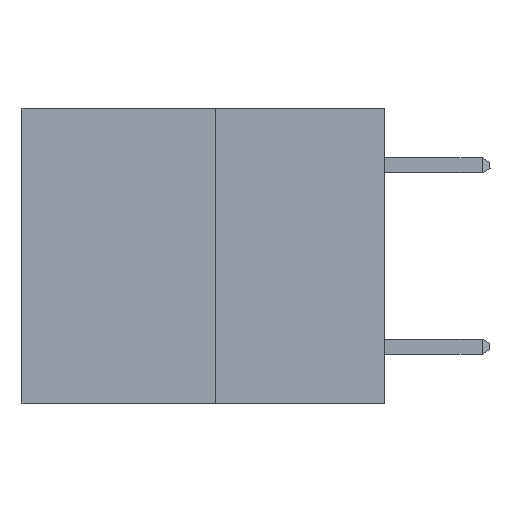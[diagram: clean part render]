
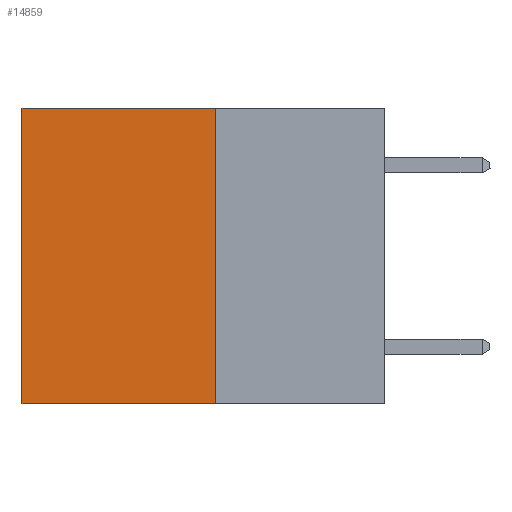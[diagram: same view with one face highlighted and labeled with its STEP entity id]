
A CAD part, left-side view. The second image highlights one B-rep face of the part: STEP entity #14859.
In plain terms, the highlighted planar face has unit normal (-1, 0, 0).
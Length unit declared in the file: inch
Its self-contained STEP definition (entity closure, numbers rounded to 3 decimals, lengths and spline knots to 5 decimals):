
#850 = DIRECTION ( 'NONE',  ( 0., 1., 0. ) ) ;
#1541 = LINE ( 'NONE', #23068, #5749 ) ;
#2603 = VECTOR ( 'NONE', #850, 39.37008 ) ;
#3437 = ORIENTED_EDGE ( 'NONE', *, *, #22030, .F. ) ;
#4077 = VECTOR ( 'NONE', #6799, 39.37008 ) ;
#4344 = VERTEX_POINT ( 'NONE', #21562 ) ;
#5150 = DIRECTION ( 'NONE',  ( 0., 0., -1. ) ) ;
#5749 = VECTOR ( 'NONE', #22993, 39.37008 ) ;
#6559 = CARTESIAN_POINT ( 'NONE',  ( 0.3165, 0.28, -0.49 ) ) ;
#6799 = DIRECTION ( 'NONE',  ( 0., 0., -1. ) ) ;
#6869 = FACE_OUTER_BOUND ( 'NONE', #19463, .T. ) ;
#7424 = AXIS2_PLACEMENT_3D ( 'NONE', #11997, #17284, #8330 ) ;
#7806 = VERTEX_POINT ( 'NONE', #21956 ) ;
#8330 = DIRECTION ( 'NONE',  ( 0., 0., -1. ) ) ;
#9907 = CARTESIAN_POINT ( 'NONE',  ( 0.3165, 0.6, -0.49 ) ) ;
#9951 = CARTESIAN_POINT ( 'NONE',  ( 0.3165, 0.6, 0. ) ) ;
#11497 = ORIENTED_EDGE ( 'NONE', *, *, #23330, .T. ) ;
#11788 = CARTESIAN_POINT ( 'NONE',  ( 0.3165, 0.28, -0.49 ) ) ;
#11997 = CARTESIAN_POINT ( 'NONE',  ( 0.3165, 0.28, -0.49 ) ) ;
#12195 = VERTEX_POINT ( 'NONE', #9951 ) ;
#12537 = ORIENTED_EDGE ( 'NONE', *, *, #13540, .T. ) ;
#13540 = EDGE_CURVE ( 'NONE', #4344, #12195, #1541, .T. ) ;
#14174 = LINE ( 'NONE', #11788, #2603 ) ;
#14859 = ADVANCED_FACE ( 'NONE', ( #6869 ), #17208, .F. ) ;
#16576 = CARTESIAN_POINT ( 'NONE',  ( 0.3165, 0.6, -0.49 ) ) ;
#17044 = ORIENTED_EDGE ( 'NONE', *, *, #20239, .F. ) ;
#17208 = PLANE ( 'NONE',  #7424 ) ;
#17284 = DIRECTION ( 'NONE',  ( 1., 0., 0. ) ) ;
#19463 = EDGE_LOOP ( 'NONE', ( #11497, #3437, #17044, #12537 ) ) ;
#20211 = LINE ( 'NONE', #6559, #4077 ) ;
#20239 = EDGE_CURVE ( 'NONE', #4344, #7806, #20211, .T. ) ;
#21172 = VECTOR ( 'NONE', #5150, 39.37008 ) ;
#21562 = CARTESIAN_POINT ( 'NONE',  ( 0.3165, 0.28, 0. ) ) ;
#21956 = CARTESIAN_POINT ( 'NONE',  ( 0.3165, 0.28, -0.49 ) ) ;
#22025 = VERTEX_POINT ( 'NONE', #16576 ) ;
#22030 = EDGE_CURVE ( 'NONE', #7806, #22025, #14174, .T. ) ;
#22993 = DIRECTION ( 'NONE',  ( 0., 1., 0. ) ) ;
#23068 = CARTESIAN_POINT ( 'NONE',  ( 0.3165, 0.28, 0. ) ) ;
#23153 = LINE ( 'NONE', #9907, #21172 ) ;
#23330 = EDGE_CURVE ( 'NONE', #12195, #22025, #23153, .T. ) ;
